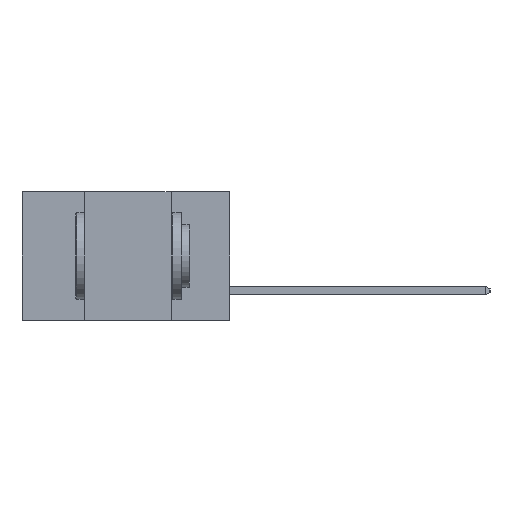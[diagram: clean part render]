
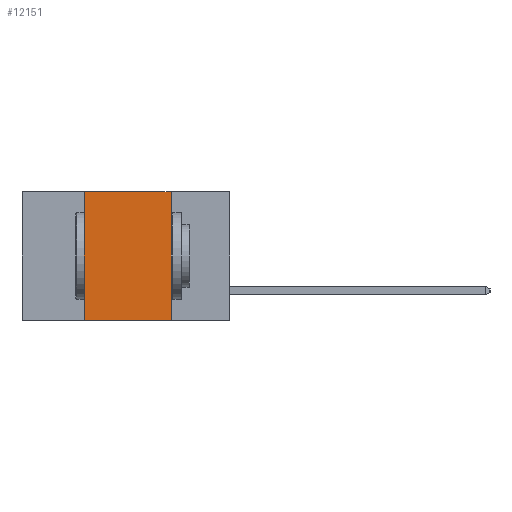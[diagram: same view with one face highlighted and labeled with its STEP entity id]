
A CAD part, left-side view. The second image highlights one B-rep face of the part: STEP entity #12151.
In plain terms, the highlighted planar face has unit normal (-1, 0, 0).
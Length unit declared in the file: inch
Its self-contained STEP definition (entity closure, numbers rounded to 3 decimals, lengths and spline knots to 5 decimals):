
#2567 = LINE ( 'NONE', #19477, #14427 ) ;
#3593 = VERTEX_POINT ( 'NONE', #15128 ) ;
#5008 = DIRECTION ( 'NONE',  ( 1., 0., 0. ) ) ;
#6128 = EDGE_CURVE ( 'NONE', #14280, #23632, #14587, .T. ) ;
#6590 = EDGE_CURVE ( 'NONE', #3593, #31185, #32250, .T. ) ;
#7617 = ORIENTED_EDGE ( 'NONE', *, *, #6128, .T. ) ;
#7829 = FACE_OUTER_BOUND ( 'NONE', #19761, .T. ) ;
#8031 = DIRECTION ( 'NONE',  ( 0., -1., 0. ) ) ;
#8549 = DIRECTION ( 'NONE',  ( 0., 0., 1. ) ) ;
#9799 = ORIENTED_EDGE ( 'NONE', *, *, #14585, .F. ) ;
#9839 = CARTESIAN_POINT ( 'NONE',  ( 0., 0.6, -0.37 ) ) ;
#11217 = ORIENTED_EDGE ( 'NONE', *, *, #6590, .F. ) ;
#12151 = ADVANCED_FACE ( 'NONE', ( #7829 ), #17611, .F. ) ;
#12188 = VECTOR ( 'NONE', #13968, 39.37008 ) ;
#13968 = DIRECTION ( 'NONE',  ( 0., -1., 0. ) ) ;
#14280 = VERTEX_POINT ( 'NONE', #32533 ) ;
#14427 = VECTOR ( 'NONE', #22004, 39.37008 ) ;
#14585 = EDGE_CURVE ( 'NONE', #14280, #3593, #25086, .T. ) ;
#14587 = LINE ( 'NONE', #9839, #28003 ) ;
#15128 = CARTESIAN_POINT ( 'NONE',  ( 0., 0.42, 0. ) ) ;
#16891 = CARTESIAN_POINT ( 'NONE',  ( 0., 0.17, 0. ) ) ;
#17611 = PLANE ( 'NONE',  #26790 ) ;
#19477 = CARTESIAN_POINT ( 'NONE',  ( 0., 0.17, 0. ) ) ;
#19761 = EDGE_LOOP ( 'NONE', ( #28257, #11217, #9799, #7617 ) ) ;
#20186 = CARTESIAN_POINT ( 'NONE',  ( 0., 0.6, 0. ) ) ;
#22004 = DIRECTION ( 'NONE',  ( 0., 0., -1. ) ) ;
#22727 = DIRECTION ( 'NONE',  ( 0., 0., -1. ) ) ;
#23085 = EDGE_CURVE ( 'NONE', #31185, #23632, #2567, .T. ) ;
#23632 = VERTEX_POINT ( 'NONE', #24062 ) ;
#24062 = CARTESIAN_POINT ( 'NONE',  ( 0., 0.17, -0.37 ) ) ;
#25086 = LINE ( 'NONE', #31325, #25270 ) ;
#25270 = VECTOR ( 'NONE', #8549, 39.37008 ) ;
#26538 = CARTESIAN_POINT ( 'NONE',  ( 0., 0.6, 0. ) ) ;
#26790 = AXIS2_PLACEMENT_3D ( 'NONE', #20186, #5008, #22727 ) ;
#28003 = VECTOR ( 'NONE', #8031, 39.37008 ) ;
#28257 = ORIENTED_EDGE ( 'NONE', *, *, #23085, .F. ) ;
#31185 = VERTEX_POINT ( 'NONE', #16891 ) ;
#31325 = CARTESIAN_POINT ( 'NONE',  ( 0., 0.42, 0. ) ) ;
#32250 = LINE ( 'NONE', #26538, #12188 ) ;
#32533 = CARTESIAN_POINT ( 'NONE',  ( 0., 0.42, -0.37 ) ) ;
